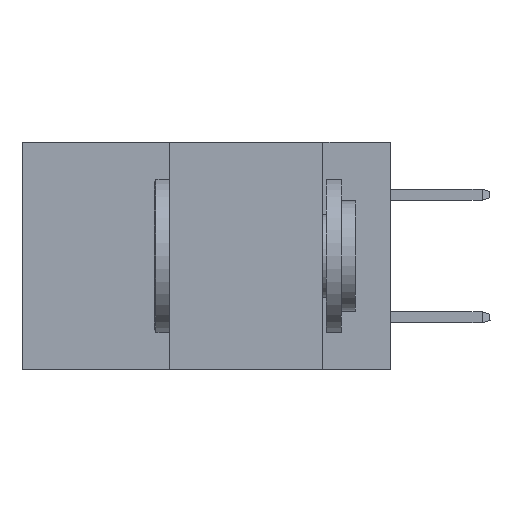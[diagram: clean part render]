
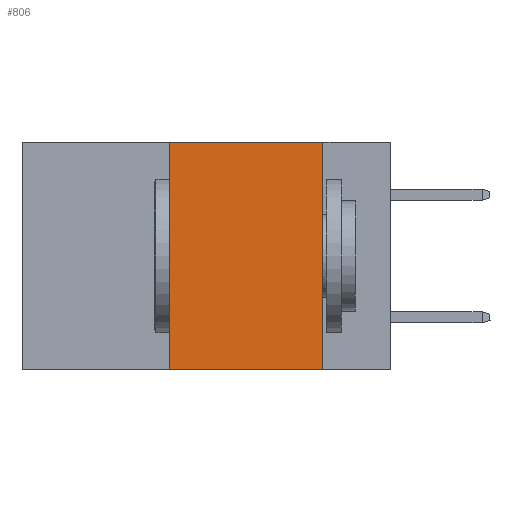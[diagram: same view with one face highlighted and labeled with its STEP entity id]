
A CAD part, left-side view. The second image highlights one B-rep face of the part: STEP entity #806.
In plain terms, the highlighted planar face has unit normal (-1, 0, 0).
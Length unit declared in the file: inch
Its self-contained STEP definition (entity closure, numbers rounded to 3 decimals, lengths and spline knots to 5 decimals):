
#806 = ADVANCED_FACE ( 'NONE', ( #3885 ), #5021, .F. ) ;
#809 = CARTESIAN_POINT ( 'NONE',  ( 0., 0.11, 0. ) ) ;
#861 = VECTOR ( 'NONE', #10538, 39.37008 ) ;
#927 = LINE ( 'NONE', #809, #4501 ) ;
#941 = VECTOR ( 'NONE', #10430, 39.37008 ) ;
#960 = LINE ( 'NONE', #15725, #941 ) ;
#1172 = VERTEX_POINT ( 'NONE', #8389 ) ;
#1529 = VERTEX_POINT ( 'NONE', #6082 ) ;
#2032 = ORIENTED_EDGE ( 'NONE', *, *, #12995, .F. ) ;
#3257 = CARTESIAN_POINT ( 'NONE',  ( 0., 0.36, -0.37 ) ) ;
#3885 = FACE_OUTER_BOUND ( 'NONE', #10009, .T. ) ;
#4123 = ORIENTED_EDGE ( 'NONE', *, *, #7741, .F. ) ;
#4501 = VECTOR ( 'NONE', #8875, 39.37008 ) ;
#4997 = DIRECTION ( 'NONE',  ( 0., -1., 0. ) ) ;
#5021 = PLANE ( 'NONE',  #16365 ) ;
#5515 = ORIENTED_EDGE ( 'NONE', *, *, #12978, .T. ) ;
#6082 = CARTESIAN_POINT ( 'NONE',  ( 0., 0.11, -0.37 ) ) ;
#6577 = ORIENTED_EDGE ( 'NONE', *, *, #7035, .F. ) ;
#7035 = EDGE_CURVE ( 'NONE', #15443, #1529, #927, .T. ) ;
#7334 = VERTEX_POINT ( 'NONE', #3257 ) ;
#7741 = EDGE_CURVE ( 'NONE', #1172, #15443, #12829, .T. ) ;
#7978 = DIRECTION ( 'NONE',  ( 0., 0., -1. ) ) ;
#8111 = CARTESIAN_POINT ( 'NONE',  ( 0., 0.11, 0. ) ) ;
#8389 = CARTESIAN_POINT ( 'NONE',  ( 0., 0.36, 0. ) ) ;
#8707 = VECTOR ( 'NONE', #4997, 39.37008 ) ;
#8875 = DIRECTION ( 'NONE',  ( 0., 0., -1. ) ) ;
#10009 = EDGE_LOOP ( 'NONE', ( #6577, #4123, #2032, #5515 ) ) ;
#10430 = DIRECTION ( 'NONE',  ( 0., -1., 0. ) ) ;
#10538 = DIRECTION ( 'NONE',  ( 0., 0., 1. ) ) ;
#12829 = LINE ( 'NONE', #16062, #8707 ) ;
#12978 = EDGE_CURVE ( 'NONE', #7334, #1529, #960, .T. ) ;
#12995 = EDGE_CURVE ( 'NONE', #7334, #1172, #14248, .T. ) ;
#13602 = CARTESIAN_POINT ( 'NONE',  ( 0., 0.6, 0. ) ) ;
#14248 = LINE ( 'NONE', #14621, #861 ) ;
#14621 = CARTESIAN_POINT ( 'NONE',  ( 0., 0.36, 0. ) ) ;
#14756 = DIRECTION ( 'NONE',  ( 1., 0., 0. ) ) ;
#15443 = VERTEX_POINT ( 'NONE', #8111 ) ;
#15725 = CARTESIAN_POINT ( 'NONE',  ( 0., 0.6, -0.37 ) ) ;
#16062 = CARTESIAN_POINT ( 'NONE',  ( 0., 0.6, 0. ) ) ;
#16365 = AXIS2_PLACEMENT_3D ( 'NONE', #13602, #14756, #7978 ) ;
